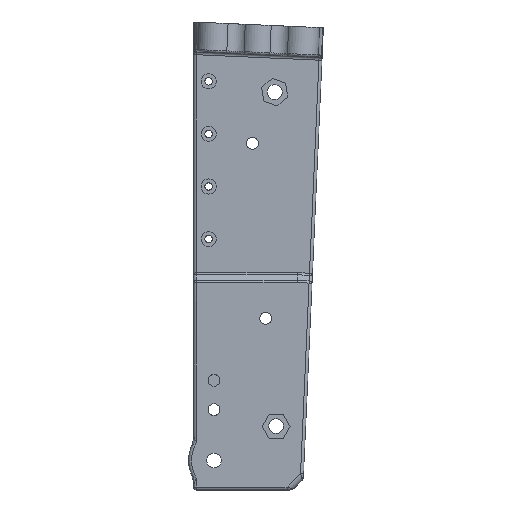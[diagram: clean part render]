
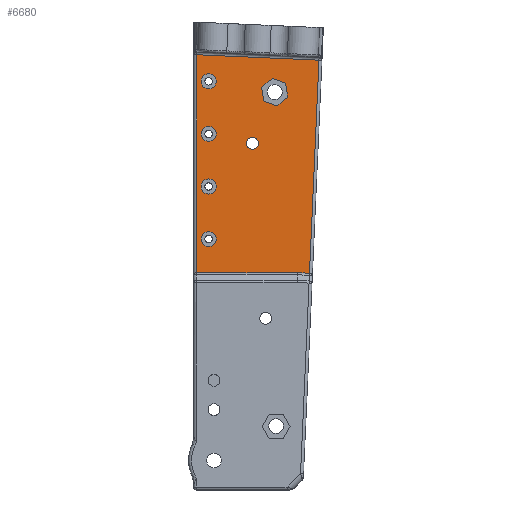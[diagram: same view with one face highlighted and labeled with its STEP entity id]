
A CAD part, left-side view. The second image highlights one B-rep face of the part: STEP entity #6680.
In plain terms, the highlighted planar face has unit normal (-1, 0, 0).
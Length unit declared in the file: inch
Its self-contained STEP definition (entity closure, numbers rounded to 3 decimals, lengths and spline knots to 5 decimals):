
#346=FACE_BOUND('',#1428,.T.);
#347=FACE_BOUND('',#1429,.T.);
#348=FACE_BOUND('',#1430,.T.);
#349=FACE_BOUND('',#1431,.T.);
#350=FACE_BOUND('',#1432,.T.);
#351=FACE_BOUND('',#1433,.T.);
#477=CIRCLE('',#7086,0.1);
#478=CIRCLE('',#7087,0.1);
#482=CIRCLE('',#7093,0.1);
#483=CIRCLE('',#7094,0.1);
#487=CIRCLE('',#7100,0.1);
#488=CIRCLE('',#7101,0.1);
#492=CIRCLE('',#7107,0.1);
#493=CIRCLE('',#7108,0.1);
#622=CIRCLE('',#7337,0.07874);
#623=CIRCLE('',#7338,0.07874);
#696=ELLIPSE('',#7288,0.11141,0.07874);
#993=FACE_OUTER_BOUND('',#1427,.T.);
#1427=EDGE_LOOP('',(#5768,#5769,#5770,#5771,#5772,#5773));
#1428=EDGE_LOOP('',(#5774,#5775,#5776,#5777,#5778,#5779));
#1429=EDGE_LOOP('',(#5780,#5781));
#1430=EDGE_LOOP('',(#5782,#5783));
#1431=EDGE_LOOP('',(#5784,#5785));
#1432=EDGE_LOOP('',(#5786,#5787));
#1433=EDGE_LOOP('',(#5788,#5789));
#1921=LINE('',#11339,#2488);
#1925=LINE('',#11347,#2492);
#1928=LINE('',#11353,#2495);
#1931=LINE('',#11359,#2498);
#1934=LINE('',#11365,#2501);
#1937=LINE('',#11370,#2504);
#1973=LINE('',#11983,#2540);
#1992=LINE('',#12574,#2559);
#1994=LINE('',#12601,#2561);
#2000=LINE('',#12635,#2567);
#2001=LINE('',#12637,#2568);
#2488=VECTOR('',#8382,0.3937);
#2492=VECTOR('',#8388,0.3937);
#2495=VECTOR('',#8393,0.3937);
#2498=VECTOR('',#8398,0.3937);
#2501=VECTOR('',#8403,0.3937);
#2504=VECTOR('',#8408,0.3937);
#2540=VECTOR('',#8726,0.3937);
#2559=VECTOR('',#8903,0.3937);
#2561=VECTOR('',#8915,0.3937);
#2567=VECTOR('',#8935,0.3937);
#2568=VECTOR('',#8938,0.3937);
#3067=VERTEX_POINT('',#11337);
#3068=VERTEX_POINT('',#11338);
#3071=VERTEX_POINT('',#11346);
#3073=VERTEX_POINT('',#11352);
#3075=VERTEX_POINT('',#11358);
#3077=VERTEX_POINT('',#11364);
#3090=VERTEX_POINT('',#11414);
#3091=VERTEX_POINT('',#11416);
#3095=VERTEX_POINT('',#11427);
#3096=VERTEX_POINT('',#11429);
#3100=VERTEX_POINT('',#11440);
#3101=VERTEX_POINT('',#11442);
#3105=VERTEX_POINT('',#11453);
#3106=VERTEX_POINT('',#11455);
#3166=VERTEX_POINT('',#11969);
#3170=VERTEX_POINT('',#11981);
#3233=VERTEX_POINT('',#12567);
#3235=VERTEX_POINT('',#12572);
#3237=VERTEX_POINT('',#12593);
#3239=VERTEX_POINT('',#12599);
#3249=VERTEX_POINT('',#12777);
#3250=VERTEX_POINT('',#12778);
#3848=EDGE_CURVE('',#3067,#3068,#1921,.T.);
#3852=EDGE_CURVE('',#3071,#3067,#1925,.T.);
#3855=EDGE_CURVE('',#3073,#3071,#1928,.T.);
#3858=EDGE_CURVE('',#3075,#3073,#1931,.T.);
#3861=EDGE_CURVE('',#3077,#3075,#1934,.T.);
#3864=EDGE_CURVE('',#3068,#3077,#1937,.T.);
#3887=EDGE_CURVE('',#3091,#3090,#477,.T.);
#3888=EDGE_CURVE('',#3090,#3091,#478,.T.);
#3893=EDGE_CURVE('',#3096,#3095,#482,.T.);
#3894=EDGE_CURVE('',#3095,#3096,#483,.T.);
#3899=EDGE_CURVE('',#3101,#3100,#487,.T.);
#3900=EDGE_CURVE('',#3100,#3101,#488,.T.);
#3905=EDGE_CURVE('',#3106,#3105,#492,.T.);
#3906=EDGE_CURVE('',#3105,#3106,#493,.T.);
#4004=EDGE_CURVE('',#3170,#3166,#1973,.T.);
#4101=EDGE_CURVE('',#3235,#3233,#1992,.T.);
#4104=EDGE_CURVE('',#3237,#3235,#696,.T.);
#4107=EDGE_CURVE('',#3239,#3237,#1994,.T.);
#4116=EDGE_CURVE('',#3233,#3170,#2000,.T.);
#4117=EDGE_CURVE('',#3166,#3239,#2001,.T.);
#4155=EDGE_CURVE('',#3249,#3250,#622,.T.);
#4156=EDGE_CURVE('',#3250,#3249,#623,.T.);
#5768=ORIENTED_EDGE('',*,*,#4004,.F.);
#5769=ORIENTED_EDGE('',*,*,#4116,.F.);
#5770=ORIENTED_EDGE('',*,*,#4101,.F.);
#5771=ORIENTED_EDGE('',*,*,#4104,.F.);
#5772=ORIENTED_EDGE('',*,*,#4107,.F.);
#5773=ORIENTED_EDGE('',*,*,#4117,.F.);
#5774=ORIENTED_EDGE('',*,*,#3848,.T.);
#5775=ORIENTED_EDGE('',*,*,#3864,.T.);
#5776=ORIENTED_EDGE('',*,*,#3861,.T.);
#5777=ORIENTED_EDGE('',*,*,#3858,.T.);
#5778=ORIENTED_EDGE('',*,*,#3855,.T.);
#5779=ORIENTED_EDGE('',*,*,#3852,.T.);
#5780=ORIENTED_EDGE('',*,*,#3887,.T.);
#5781=ORIENTED_EDGE('',*,*,#3888,.T.);
#5782=ORIENTED_EDGE('',*,*,#3893,.T.);
#5783=ORIENTED_EDGE('',*,*,#3894,.T.);
#5784=ORIENTED_EDGE('',*,*,#3899,.T.);
#5785=ORIENTED_EDGE('',*,*,#3900,.T.);
#5786=ORIENTED_EDGE('',*,*,#3905,.T.);
#5787=ORIENTED_EDGE('',*,*,#3906,.T.);
#5788=ORIENTED_EDGE('',*,*,#4155,.T.);
#5789=ORIENTED_EDGE('',*,*,#4156,.T.);
#6342=PLANE('',#7336);
#6680=ADVANCED_FACE('',(#993,#346,#347,#348,#349,#350,#351),#6342,.F.);
#7086=AXIS2_PLACEMENT_3D('',#11417,#8461,#8462);
#7087=AXIS2_PLACEMENT_3D('',#11418,#8463,#8464);
#7093=AXIS2_PLACEMENT_3D('',#11430,#8476,#8477);
#7094=AXIS2_PLACEMENT_3D('',#11431,#8478,#8479);
#7100=AXIS2_PLACEMENT_3D('',#11443,#8491,#8492);
#7101=AXIS2_PLACEMENT_3D('',#11444,#8493,#8494);
#7107=AXIS2_PLACEMENT_3D('',#11456,#8506,#8507);
#7108=AXIS2_PLACEMENT_3D('',#11457,#8508,#8509);
#7288=AXIS2_PLACEMENT_3D('',#12595,#8907,#8908);
#7336=AXIS2_PLACEMENT_3D('',#12776,#9040,#9041);
#7337=AXIS2_PLACEMENT_3D('',#12779,#9042,#9043);
#7338=AXIS2_PLACEMENT_3D('',#12780,#9044,#9045);
#8382=DIRECTION('',(0.,0.153,0.988));
#8388=DIRECTION('',(0.,0.932,0.362));
#8393=DIRECTION('',(0.,0.78,-0.626));
#8398=DIRECTION('',(0.,-0.153,-0.988));
#8403=DIRECTION('',(0.,-0.932,-0.362));
#8408=DIRECTION('',(0.,-0.78,0.626));
#8461=DIRECTION('center_axis',(1.,0.,0.));
#8462=DIRECTION('ref_axis',(0.,0.,-1.));
#8463=DIRECTION('center_axis',(1.,0.,0.));
#8464=DIRECTION('ref_axis',(0.,0.,-1.));
#8476=DIRECTION('center_axis',(1.,0.,0.));
#8477=DIRECTION('ref_axis',(0.,0.,-1.));
#8478=DIRECTION('center_axis',(1.,0.,0.));
#8479=DIRECTION('ref_axis',(0.,0.,-1.));
#8491=DIRECTION('center_axis',(1.,0.,0.));
#8492=DIRECTION('ref_axis',(0.,0.,-1.));
#8493=DIRECTION('center_axis',(1.,0.,0.));
#8494=DIRECTION('ref_axis',(0.,0.,-1.));
#8506=DIRECTION('center_axis',(1.,0.,0.));
#8507=DIRECTION('ref_axis',(0.,0.,-1.));
#8508=DIRECTION('center_axis',(1.,0.,0.));
#8509=DIRECTION('ref_axis',(0.,0.,-1.));
#8726=DIRECTION('',(0.,-0.999,-0.044));
#8903=DIRECTION('',(0.,1.,0.));
#8907=DIRECTION('center_axis',(-1.,0.,0.));
#8908=DIRECTION('ref_axis',(0.,-0.044,0.999));
#8915=DIRECTION('',(0.,0.999,0.044));
#8935=DIRECTION('',(0.,0.,1.));
#8938=DIRECTION('',(0.,0.044,-0.999));
#9040=DIRECTION('center_axis',(1.,0.,0.));
#9041=DIRECTION('ref_axis',(0.,0.,-1.));
#9042=DIRECTION('center_axis',(1.,0.,0.));
#9043=DIRECTION('ref_axis',(0.,0.,1.));
#9044=DIRECTION('center_axis',(1.,0.,0.));
#9045=DIRECTION('ref_axis',(0.,0.,1.));
#11337=CARTESIAN_POINT('',(-1.06693,-0.93739,5.17852));
#11338=CARTESIAN_POINT('',(-1.06693,-0.90892,5.36273));
#11339=CARTESIAN_POINT('',(-1.06693,-0.99565,4.80145));
#11346=CARTESIAN_POINT('',(-1.06693,-1.11114,5.11107));
#11347=CARTESIAN_POINT('',(-1.06693,-1.1258,5.10538));
#11352=CARTESIAN_POINT('',(-1.06693,-1.25643,5.22782));
#11353=CARTESIAN_POINT('',(-1.06693,-0.93495,4.96949));
#11358=CARTESIAN_POINT('',(-1.06693,-1.22797,5.41203));
#11359=CARTESIAN_POINT('',(-1.06693,-1.30047,4.94285));
#11364=CARTESIAN_POINT('',(-1.06693,-1.05421,5.47948));
#11365=CARTESIAN_POINT('',(-1.06693,-1.15575,5.44006));
#11370=CARTESIAN_POINT('',(-1.06693,-0.66008,5.16277));
#11414=CARTESIAN_POINT('',(-1.06693,-0.20416,4.13881));
#11416=CARTESIAN_POINT('',(-1.06693,-0.20416,3.93881));
#11417=CARTESIAN_POINT('Origin',(-1.06693,-0.20416,4.03881));
#11418=CARTESIAN_POINT('Origin',(-1.06693,-0.20416,4.03881));
#11427=CARTESIAN_POINT('',(-1.06693,-0.20416,4.83881));
#11429=CARTESIAN_POINT('',(-1.06693,-0.20416,4.63881));
#11430=CARTESIAN_POINT('Origin',(-1.06693,-0.20416,4.73881));
#11431=CARTESIAN_POINT('Origin',(-1.06693,-0.20416,4.73881));
#11440=CARTESIAN_POINT('',(-1.06693,-0.20416,3.43881));
#11442=CARTESIAN_POINT('',(-1.06693,-0.20416,3.23881));
#11443=CARTESIAN_POINT('Origin',(-1.06693,-0.20416,3.33881));
#11444=CARTESIAN_POINT('Origin',(-1.06693,-0.20416,3.33881));
#11453=CARTESIAN_POINT('',(-1.06693,-0.20416,5.53881));
#11455=CARTESIAN_POINT('',(-1.06693,-0.20416,5.33881));
#11456=CARTESIAN_POINT('Origin',(-1.06693,-0.20416,5.43881));
#11457=CARTESIAN_POINT('Origin',(-1.06693,-0.20416,5.43881));
#11969=CARTESIAN_POINT('',(-1.06693,-1.67223,5.7202));
#11981=CARTESIAN_POINT('',(-1.06693,-0.04275,5.79277));
#11983=CARTESIAN_POINT('',(-1.06693,-0.88771,5.75514));
#12567=CARTESIAN_POINT('',(-1.06693,-0.04275,2.89196));
#12572=CARTESIAN_POINT('',(-1.06693,-1.38678,2.89196));
#12574=CARTESIAN_POINT('',(-1.06693,-0.4344,2.89196));
#12593=CARTESIAN_POINT('',(-1.06693,-1.38925,2.89191));
#12595=CARTESIAN_POINT('Origin',(-1.06693,-1.3843,2.78061));
#12599=CARTESIAN_POINT('',(-1.06693,-1.54596,2.88493));
#12601=CARTESIAN_POINT('',(-1.06693,-1.09497,2.90501));
#12635=CARTESIAN_POINT('',(-1.06693,-0.04275,2.19775));
#12637=CARTESIAN_POINT('',(-1.06693,-1.56451,3.30156));
#12776=CARTESIAN_POINT('Origin',(-1.06693,-0.8671,4.39551));
#12777=CARTESIAN_POINT('',(-1.06693,-0.7874,4.53543));
#12778=CARTESIAN_POINT('',(-1.06693,-0.7874,4.69291));
#12779=CARTESIAN_POINT('Origin',(-1.06693,-0.7874,4.61417));
#12780=CARTESIAN_POINT('Origin',(-1.06693,-0.7874,4.61417));
